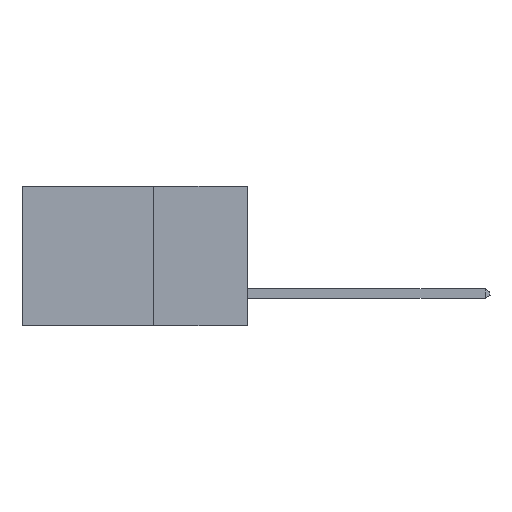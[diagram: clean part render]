
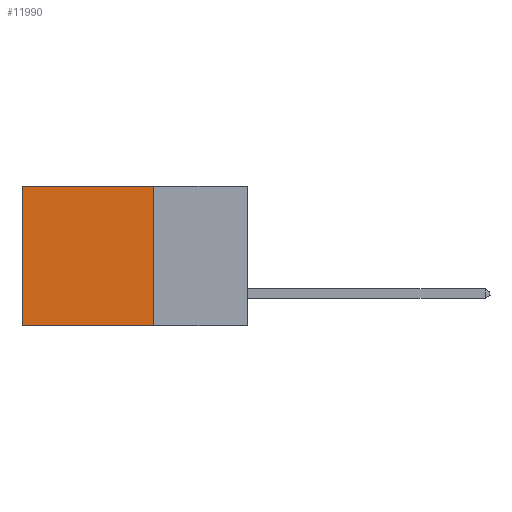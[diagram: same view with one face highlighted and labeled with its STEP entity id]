
A CAD part, left-side view. The second image highlights one B-rep face of the part: STEP entity #11990.
In plain terms, the highlighted planar face has unit normal (-1, 0, 0).
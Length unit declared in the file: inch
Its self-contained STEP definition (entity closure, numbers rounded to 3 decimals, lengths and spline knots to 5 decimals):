
#612 = DIRECTION ( 'NONE',  ( 0., 0., -1. ) ) ;
#1322 = ORIENTED_EDGE ( 'NONE', *, *, #7015, .T. ) ;
#1430 = VECTOR ( 'NONE', #2402, 39.37008 ) ;
#2402 = DIRECTION ( 'NONE',  ( 0., 1., 0. ) ) ;
#2518 = ORIENTED_EDGE ( 'NONE', *, *, #19281, .T. ) ;
#2836 = CARTESIAN_POINT ( 'NONE',  ( 0.298, 0.6, 0. ) ) ;
#3779 = CARTESIAN_POINT ( 'NONE',  ( 0.298, 0.6, 0. ) ) ;
#3970 = PLANE ( 'NONE',  #14101 ) ;
#4019 = VECTOR ( 'NONE', #6884, 39.37008 ) ;
#5078 = CARTESIAN_POINT ( 'NONE',  ( 0.298, 0.25, -0.37 ) ) ;
#5111 = EDGE_CURVE ( 'NONE', #9433, #8474, #6989, .T. ) ;
#5246 = CARTESIAN_POINT ( 'NONE',  ( 0.298, 0.25, 0. ) ) ;
#5255 = VERTEX_POINT ( 'NONE', #2836 ) ;
#5548 = LINE ( 'NONE', #5246, #1430 ) ;
#5731 = EDGE_LOOP ( 'NONE', ( #2518, #6762, #7451, #1322 ) ) ;
#6270 = LINE ( 'NONE', #9505, #17039 ) ;
#6762 = ORIENTED_EDGE ( 'NONE', *, *, #5111, .F. ) ;
#6884 = DIRECTION ( 'NONE',  ( 0., 1., 0. ) ) ;
#6989 = LINE ( 'NONE', #8465, #4019 ) ;
#7015 = EDGE_CURVE ( 'NONE', #16388, #5255, #5548, .T. ) ;
#7451 = ORIENTED_EDGE ( 'NONE', *, *, #10869, .F. ) ;
#8175 = LINE ( 'NONE', #3779, #20112 ) ;
#8465 = CARTESIAN_POINT ( 'NONE',  ( 0.298, 0.25, -0.37 ) ) ;
#8474 = VERTEX_POINT ( 'NONE', #12465 ) ;
#9433 = VERTEX_POINT ( 'NONE', #5078 ) ;
#9505 = CARTESIAN_POINT ( 'NONE',  ( 0.298, 0.25, 0. ) ) ;
#9605 = CARTESIAN_POINT ( 'NONE',  ( 0.298, 0.25, 0. ) ) ;
#10134 = DIRECTION ( 'NONE',  ( 0., 0., -1. ) ) ;
#10281 = CARTESIAN_POINT ( 'NONE',  ( 0.298, 0.25, 0. ) ) ;
#10869 = EDGE_CURVE ( 'NONE', #16388, #9433, #6270, .T. ) ;
#11748 = DIRECTION ( 'NONE',  ( 1., 0., 0. ) ) ;
#11990 = ADVANCED_FACE ( 'NONE', ( #19575 ), #3970, .F. ) ;
#12465 = CARTESIAN_POINT ( 'NONE',  ( 0.298, 0.6, -0.37 ) ) ;
#13928 = DIRECTION ( 'NONE',  ( 0., 0., -1. ) ) ;
#14101 = AXIS2_PLACEMENT_3D ( 'NONE', #10281, #11748, #10134 ) ;
#16388 = VERTEX_POINT ( 'NONE', #9605 ) ;
#17039 = VECTOR ( 'NONE', #13928, 39.37008 ) ;
#19281 = EDGE_CURVE ( 'NONE', #5255, #8474, #8175, .T. ) ;
#19575 = FACE_OUTER_BOUND ( 'NONE', #5731, .T. ) ;
#20112 = VECTOR ( 'NONE', #612, 39.37008 ) ;
